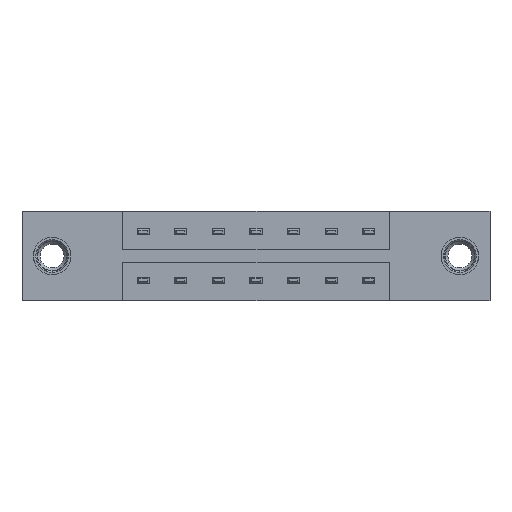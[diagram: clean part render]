
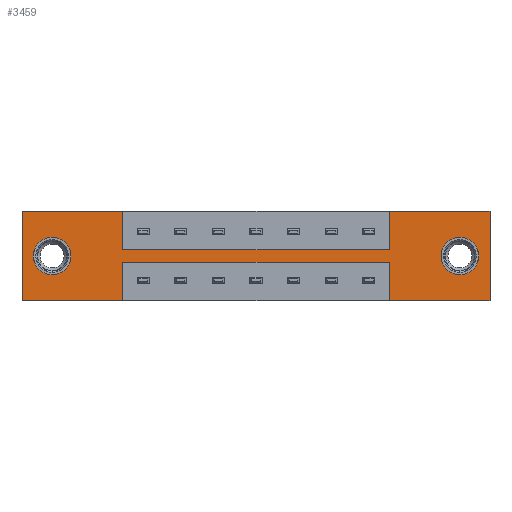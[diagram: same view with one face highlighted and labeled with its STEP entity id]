
A CAD part, front view. The second image highlights one B-rep face of the part: STEP entity #3459.
In plain terms, the highlighted planar face has unit normal (0, -1, 0).
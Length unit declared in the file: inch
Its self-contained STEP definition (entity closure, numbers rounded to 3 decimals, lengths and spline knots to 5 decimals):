
#126 = CARTESIAN_POINT ( 'NONE',  ( 1.5225, 0., -0.1585 ) ) ;
#248 = CARTESIAN_POINT ( 'NONE',  ( 1.94, 0., 0. ) ) ;
#289 = ORIENTED_EDGE ( 'NONE', *, *, #4080, .F. ) ;
#349 = CARTESIAN_POINT ( 'NONE',  ( 0.4175, 0., -0.2115 ) ) ;
#467 = VECTOR ( 'NONE', #8524, 39.37008 ) ;
#558 = CARTESIAN_POINT ( 'NONE',  ( 0.4175, 0., -0.37 ) ) ;
#590 = CARTESIAN_POINT ( 'NONE',  ( 1.94, 0., 0. ) ) ;
#846 = CARTESIAN_POINT ( 'NONE',  ( 1.5225, 0., -0.37 ) ) ;
#1026 = CARTESIAN_POINT ( 'NONE',  ( 1.815, 0., -0.107 ) ) ;
#1086 = CARTESIAN_POINT ( 'NONE',  ( 0., 0., -0.37 ) ) ;
#1143 = CARTESIAN_POINT ( 'NONE',  ( 0., 0., -0.37 ) ) ;
#1222 = ORIENTED_EDGE ( 'NONE', *, *, #7026, .T. ) ;
#1260 = CARTESIAN_POINT ( 'NONE',  ( 0., 0., 0. ) ) ;
#1354 = CARTESIAN_POINT ( 'NONE',  ( 0., 0., 0. ) ) ;
#1371 = DIRECTION ( 'NONE',  ( 0., 1., 0. ) ) ;
#1393 = ORIENTED_EDGE ( 'NONE', *, *, #6330, .F. ) ;
#1419 = LINE ( 'NONE', #4506, #7630 ) ;
#1437 = DIRECTION ( 'NONE',  ( 0., 1., 0. ) ) ;
#1470 = DIRECTION ( 'NONE',  ( -1., 0., 0. ) ) ;
#1544 = EDGE_CURVE ( 'NONE', #3844, #1650, #1903, .T. ) ;
#1591 = CARTESIAN_POINT ( 'NONE',  ( 0.4175, 0., -0.2115 ) ) ;
#1624 = AXIS2_PLACEMENT_3D ( 'NONE', #7693, #1437, #9752 ) ;
#1650 = VERTEX_POINT ( 'NONE', #3674 ) ;
#1659 = CARTESIAN_POINT ( 'NONE',  ( 0., 0., -0.37 ) ) ;
#1663 = VERTEX_POINT ( 'NONE', #8159 ) ;
#1846 = DIRECTION ( 'NONE',  ( 0., -1., 0. ) ) ;
#1898 = ORIENTED_EDGE ( 'NONE', *, *, #1544, .F. ) ;
#1903 = LINE ( 'NONE', #7908, #9195 ) ;
#1938 = ORIENTED_EDGE ( 'NONE', *, *, #9188, .F. ) ;
#2071 = CARTESIAN_POINT ( 'NONE',  ( 0.125, 0., -0.185 ) ) ;
#2217 = DIRECTION ( 'NONE',  ( 0., 0., 1. ) ) ;
#2442 = CARTESIAN_POINT ( 'NONE',  ( 0.4175, 0., -0.1585 ) ) ;
#2536 = VERTEX_POINT ( 'NONE', #248 ) ;
#2555 = EDGE_CURVE ( 'NONE', #1663, #6926, #4158, .T. ) ;
#2614 = FACE_OUTER_BOUND ( 'NONE', #8977, .T. ) ;
#2625 = CARTESIAN_POINT ( 'NONE',  ( 0.125, 0., -0.107 ) ) ;
#2654 = EDGE_CURVE ( 'NONE', #6784, #9602, #5215, .T. ) ;
#2759 = CARTESIAN_POINT ( 'NONE',  ( 0.125, 0., -0.185 ) ) ;
#2904 = VECTOR ( 'NONE', #3228, 39.37008 ) ;
#2998 = VERTEX_POINT ( 'NONE', #2625 ) ;
#3215 = DIRECTION ( 'NONE',  ( 1., 0., 0. ) ) ;
#3228 = DIRECTION ( 'NONE',  ( 0., 0., 1. ) ) ;
#3293 = VECTOR ( 'NONE', #4996, 39.37008 ) ;
#3315 = FACE_BOUND ( 'NONE', #3707, .T. ) ;
#3402 = AXIS2_PLACEMENT_3D ( 'NONE', #2071, #10001, #2217 ) ;
#3454 = CARTESIAN_POINT ( 'NONE',  ( 1.94, 0., -0.37 ) ) ;
#3459 = ADVANCED_FACE ( 'NONE', ( #9580, #3315, #2614 ), #5716, .T. ) ;
#3501 = EDGE_CURVE ( 'NONE', #2998, #8941, #9723, .T. ) ;
#3577 = EDGE_CURVE ( 'NONE', #2536, #6193, #7761, .T. ) ;
#3597 = LINE ( 'NONE', #349, #3916 ) ;
#3674 = CARTESIAN_POINT ( 'NONE',  ( 1.5225, 0., -0.2115 ) ) ;
#3676 = LINE ( 'NONE', #1354, #9381 ) ;
#3707 = EDGE_LOOP ( 'NONE', ( #8730, #6771 ) ) ;
#3731 = EDGE_CURVE ( 'NONE', #5620, #4317, #8015, .T. ) ;
#3844 = VERTEX_POINT ( 'NONE', #846 ) ;
#3916 = VECTOR ( 'NONE', #7418, 39.37008 ) ;
#3975 = CARTESIAN_POINT ( 'NONE',  ( 0.4175, 0., -0.1585 ) ) ;
#4080 = EDGE_CURVE ( 'NONE', #4317, #2536, #3676, .T. ) ;
#4158 = LINE ( 'NONE', #2442, #9382 ) ;
#4231 = CARTESIAN_POINT ( 'NONE',  ( 0., 0., -0.37 ) ) ;
#4317 = VERTEX_POINT ( 'NONE', #9732 ) ;
#4320 = DIRECTION ( 'NONE',  ( 0., 0., 1. ) ) ;
#4343 = VECTOR ( 'NONE', #7884, 39.37008 ) ;
#4506 = CARTESIAN_POINT ( 'NONE',  ( 0.4175, 0., -0.2115 ) ) ;
#4695 = EDGE_CURVE ( 'NONE', #9602, #1663, #5601, .T. ) ;
#4771 = ORIENTED_EDGE ( 'NONE', *, *, #8429, .F. ) ;
#4915 = CARTESIAN_POINT ( 'NONE',  ( 0.4175, 0., -0.1585 ) ) ;
#4939 = ORIENTED_EDGE ( 'NONE', *, *, #2555, .F. ) ;
#4996 = DIRECTION ( 'NONE',  ( -1., 0., 0. ) ) ;
#5145 = LINE ( 'NONE', #4231, #6810 ) ;
#5215 = LINE ( 'NONE', #1260, #6125 ) ;
#5326 = ORIENTED_EDGE ( 'NONE', *, *, #9352, .F. ) ;
#5601 = LINE ( 'NONE', #6308, #4343 ) ;
#5620 = VERTEX_POINT ( 'NONE', #8919 ) ;
#5664 = EDGE_CURVE ( 'NONE', #6193, #3844, #5145, .T. ) ;
#5716 = PLANE ( 'NONE',  #8578 ) ;
#6016 = ORIENTED_EDGE ( 'NONE', *, *, #3731, .F. ) ;
#6125 = VECTOR ( 'NONE', #9901, 39.37008 ) ;
#6193 = VERTEX_POINT ( 'NONE', #3454 ) ;
#6266 = VERTEX_POINT ( 'NONE', #558 ) ;
#6308 = CARTESIAN_POINT ( 'NONE',  ( 0., 0., 0. ) ) ;
#6330 = EDGE_CURVE ( 'NONE', #1650, #8997, #1419, .T. ) ;
#6631 = EDGE_CURVE ( 'NONE', #8941, #2998, #8280, .T. ) ;
#6661 = EDGE_CURVE ( 'NONE', #8297, #7315, #6823, .T. ) ;
#6686 = DIRECTION ( 'NONE',  ( -1., 0., 0. ) ) ;
#6714 = DIRECTION ( 'NONE',  ( 0., 0., -1. ) ) ;
#6715 = ORIENTED_EDGE ( 'NONE', *, *, #4695, .F. ) ;
#6771 = ORIENTED_EDGE ( 'NONE', *, *, #6631, .T. ) ;
#6784 = VERTEX_POINT ( 'NONE', #1659 ) ;
#6810 = VECTOR ( 'NONE', #6686, 39.37008 ) ;
#6823 = CIRCLE ( 'NONE', #9418, 0.078 ) ;
#6926 = VERTEX_POINT ( 'NONE', #4915 ) ;
#6937 = CARTESIAN_POINT ( 'NONE',  ( 0.125, 0., -0.263 ) ) ;
#7026 = EDGE_CURVE ( 'NONE', #7315, #8297, #9909, .T. ) ;
#7298 = LINE ( 'NONE', #3975, #9950 ) ;
#7315 = VERTEX_POINT ( 'NONE', #9722 ) ;
#7323 = ORIENTED_EDGE ( 'NONE', *, *, #3577, .F. ) ;
#7343 = LINE ( 'NONE', #1143, #3293 ) ;
#7418 = DIRECTION ( 'NONE',  ( 0., 0., -1. ) ) ;
#7630 = VECTOR ( 'NONE', #1470, 39.37008 ) ;
#7693 = CARTESIAN_POINT ( 'NONE',  ( 1.815, 0., -0.185 ) ) ;
#7761 = LINE ( 'NONE', #590, #467 ) ;
#7880 = DIRECTION ( 'NONE',  ( 0., 0., -1. ) ) ;
#7884 = DIRECTION ( 'NONE',  ( 1., 0., 0. ) ) ;
#7908 = CARTESIAN_POINT ( 'NONE',  ( 1.5225, 0., -0.2115 ) ) ;
#7930 = AXIS2_PLACEMENT_3D ( 'NONE', #2759, #9730, #4320 ) ;
#8015 = LINE ( 'NONE', #126, #2904 ) ;
#8159 = CARTESIAN_POINT ( 'NONE',  ( 0.4175, 0., 0. ) ) ;
#8280 = CIRCLE ( 'NONE', #3402, 0.078 ) ;
#8297 = VERTEX_POINT ( 'NONE', #1026 ) ;
#8429 = EDGE_CURVE ( 'NONE', #8997, #6266, #3597, .T. ) ;
#8524 = DIRECTION ( 'NONE',  ( 0., 0., -1. ) ) ;
#8578 = AXIS2_PLACEMENT_3D ( 'NONE', #1086, #1846, #8813 ) ;
#8678 = EDGE_LOOP ( 'NONE', ( #9549, #1222 ) ) ;
#8730 = ORIENTED_EDGE ( 'NONE', *, *, #3501, .T. ) ;
#8771 = ORIENTED_EDGE ( 'NONE', *, *, #2654, .F. ) ;
#8773 = DIRECTION ( 'NONE',  ( 0., 0., 1. ) ) ;
#8813 = DIRECTION ( 'NONE',  ( 0., 0., -1. ) ) ;
#8919 = CARTESIAN_POINT ( 'NONE',  ( 1.5225, 0., -0.1585 ) ) ;
#8941 = VERTEX_POINT ( 'NONE', #6937 ) ;
#8977 = EDGE_LOOP ( 'NONE', ( #1898, #9640, #7323, #289, #6016, #1938, #4939, #6715, #8771, #5326, #4771, #1393 ) ) ;
#8997 = VERTEX_POINT ( 'NONE', #1591 ) ;
#9186 = CARTESIAN_POINT ( 'NONE',  ( 1.815, 0., -0.185 ) ) ;
#9188 = EDGE_CURVE ( 'NONE', #6926, #5620, #7298, .T. ) ;
#9195 = VECTOR ( 'NONE', #8773, 39.37008 ) ;
#9276 = DIRECTION ( 'NONE',  ( 1., 0., 0. ) ) ;
#9352 = EDGE_CURVE ( 'NONE', #6266, #6784, #7343, .T. ) ;
#9381 = VECTOR ( 'NONE', #9276, 39.37008 ) ;
#9382 = VECTOR ( 'NONE', #7880, 39.37008 ) ;
#9413 = CARTESIAN_POINT ( 'NONE',  ( 0., 0., 0. ) ) ;
#9418 = AXIS2_PLACEMENT_3D ( 'NONE', #9186, #1371, #6714 ) ;
#9549 = ORIENTED_EDGE ( 'NONE', *, *, #6661, .T. ) ;
#9580 = FACE_BOUND ( 'NONE', #8678, .T. ) ;
#9602 = VERTEX_POINT ( 'NONE', #9413 ) ;
#9640 = ORIENTED_EDGE ( 'NONE', *, *, #5664, .F. ) ;
#9722 = CARTESIAN_POINT ( 'NONE',  ( 1.815, 0., -0.263 ) ) ;
#9723 = CIRCLE ( 'NONE', #7930, 0.078 ) ;
#9730 = DIRECTION ( 'NONE',  ( 0., 1., 0. ) ) ;
#9732 = CARTESIAN_POINT ( 'NONE',  ( 1.5225, 0., 0. ) ) ;
#9752 = DIRECTION ( 'NONE',  ( 0., 0., -1. ) ) ;
#9901 = DIRECTION ( 'NONE',  ( 0., 0., 1. ) ) ;
#9909 = CIRCLE ( 'NONE', #1624, 0.078 ) ;
#9950 = VECTOR ( 'NONE', #3215, 39.37008 ) ;
#10001 = DIRECTION ( 'NONE',  ( 0., 1., 0. ) ) ;
